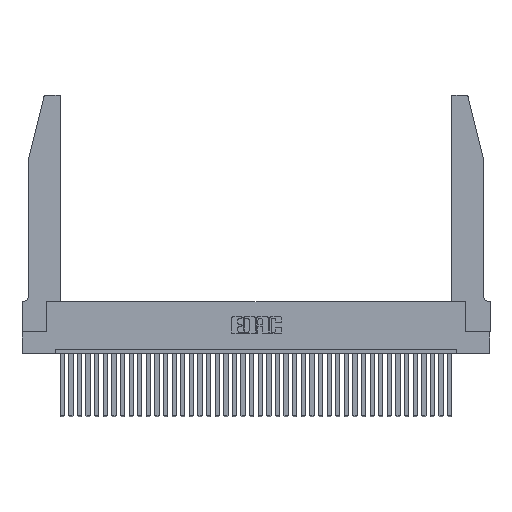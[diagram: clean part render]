
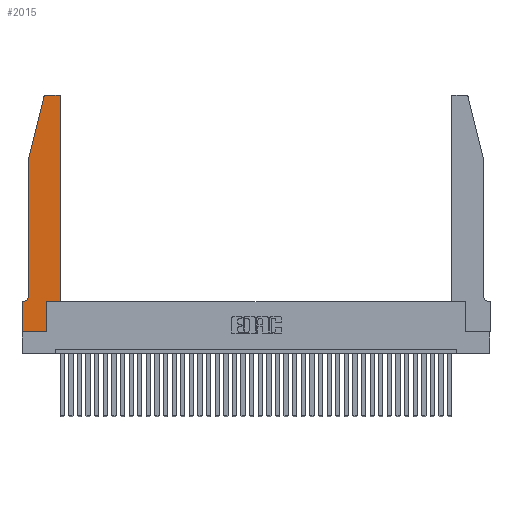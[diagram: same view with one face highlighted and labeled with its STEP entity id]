
A CAD part, top view. The second image highlights one B-rep face of the part: STEP entity #2015.
In plain terms, the highlighted planar face has unit normal (0, 0, 1).
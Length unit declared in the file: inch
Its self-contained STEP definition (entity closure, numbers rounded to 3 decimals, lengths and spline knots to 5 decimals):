
#1285 = DIRECTION ( 'NONE',  ( 0., 1., 0. ) ) ;
#1753 = DIRECTION ( 'NONE',  ( 0., 0., 1. ) ) ;
#1791 = DIRECTION ( 'NONE',  ( 0., 0., 1. ) ) ;
#1822 = EDGE_CURVE ( 'NONE', #13608, #14157, #12460, .T. ) ;
#2015 = ADVANCED_FACE ( 'NONE', ( #34438 ), #25638, .T. ) ;
#2918 = EDGE_CURVE ( 'NONE', #18267, #20375, #23190, .T. ) ;
#3709 = VECTOR ( 'NONE', #16268, 39.37008 ) ;
#4026 = CARTESIAN_POINT ( 'NONE',  ( 0.0755, 0.35, 0.37 ) ) ;
#4498 = DIRECTION ( 'NONE',  ( 1., 0., 0. ) ) ;
#4522 = DIRECTION ( 'NONE',  ( 0., 0., -1. ) ) ;
#5062 = VECTOR ( 'NONE', #18837, 39.37008 ) ;
#5622 = DIRECTION ( 'NONE',  ( 0., -1., 0. ) ) ;
#5947 = EDGE_LOOP ( 'NONE', ( #38282, #24160, #25649, #17477, #10023, #28996, #31484, #28924, #35557, #20605, #14406, #19811 ) ) ;
#6804 = CARTESIAN_POINT ( 'NONE',  ( 0., 0., 0.37 ) ) ;
#6936 = CARTESIAN_POINT ( 'NONE',  ( 0.0755, 2., 0.37 ) ) ;
#7409 = CARTESIAN_POINT ( 'NONE',  ( 0., 0., 0.37 ) ) ;
#7529 = DIRECTION ( 'NONE',  ( -1., 0., 0. ) ) ;
#7593 = DIRECTION ( 'NONE',  ( 0., 1., 0. ) ) ;
#8099 = EDGE_CURVE ( 'NONE', #35104, #13608, #25233, .T. ) ;
#8484 = CARTESIAN_POINT ( 'NONE',  ( 0.4505, 2.72, 0.37 ) ) ;
#9464 = VECTOR ( 'NONE', #1285, 39.37008 ) ;
#9716 = LINE ( 'NONE', #6936, #35869 ) ;
#10023 = ORIENTED_EDGE ( 'NONE', *, *, #11537, .T. ) ;
#10284 = VECTOR ( 'NONE', #16960, 39.37008 ) ;
#10951 = CARTESIAN_POINT ( 'NONE',  ( 0.2605, 2.75, 0.37 ) ) ;
#11537 = EDGE_CURVE ( 'NONE', #20375, #23729, #20236, .T. ) ;
#11818 = VERTEX_POINT ( 'NONE', #37445 ) ;
#12088 = CARTESIAN_POINT ( 'NONE',  ( 0.0755, 0.42, 0.37 ) ) ;
#12460 = LINE ( 'NONE', #6804, #5062 ) ;
#12712 = LINE ( 'NONE', #4026, #26757 ) ;
#13359 = CARTESIAN_POINT ( 'NONE',  ( 0.0055, 0.42, 0.37 ) ) ;
#13608 = VERTEX_POINT ( 'NONE', #33787 ) ;
#13992 = CARTESIAN_POINT ( 'NONE',  ( 0., 0.35, 0.37 ) ) ;
#14157 = VERTEX_POINT ( 'NONE', #16720 ) ;
#14386 = EDGE_CURVE ( 'NONE', #24438, #18267, #9716, .T. ) ;
#14406 = ORIENTED_EDGE ( 'NONE', *, *, #36901, .T. ) ;
#15849 = EDGE_CURVE ( 'NONE', #14157, #19823, #26891, .T. ) ;
#15952 = LINE ( 'NONE', #25290, #9464 ) ;
#16251 = EDGE_CURVE ( 'NONE', #17845, #26636, #37986, .T. ) ;
#16268 = DIRECTION ( 'NONE',  ( 1., 0., 0. ) ) ;
#16474 = DIRECTION ( 'NONE',  ( -0.239, -0.971, 0. ) ) ;
#16720 = CARTESIAN_POINT ( 'NONE',  ( 0.2865, 0., 0.37 ) ) ;
#16960 = DIRECTION ( 'NONE',  ( 0., -1., 0. ) ) ;
#17477 = ORIENTED_EDGE ( 'NONE', *, *, #2918, .T. ) ;
#17845 = VERTEX_POINT ( 'NONE', #8484 ) ;
#18103 = EDGE_CURVE ( 'NONE', #19823, #11818, #18673, .T. ) ;
#18267 = VERTEX_POINT ( 'NONE', #22051 ) ;
#18673 = LINE ( 'NONE', #28291, #3709 ) ;
#18837 = DIRECTION ( 'NONE',  ( 1., 0., 0. ) ) ;
#19685 = CARTESIAN_POINT ( 'NONE',  ( 0.4205, 2.72, 0.37 ) ) ;
#19811 = ORIENTED_EDGE ( 'NONE', *, *, #16251, .T. ) ;
#19823 = VERTEX_POINT ( 'NONE', #34626 ) ;
#19906 = DIRECTION ( 'NONE',  ( 1., 0., 0. ) ) ;
#20236 = CIRCLE ( 'NONE', #37828, 0.07 ) ;
#20375 = VERTEX_POINT ( 'NONE', #12088 ) ;
#20605 = ORIENTED_EDGE ( 'NONE', *, *, #18103, .T. ) ;
#21017 = VECTOR ( 'NONE', #31391, 39.37008 ) ;
#21255 = AXIS2_PLACEMENT_3D ( 'NONE', #37382, #1753, #4498 ) ;
#21536 = CARTESIAN_POINT ( 'NONE',  ( 0., 0.35, 0.37 ) ) ;
#22051 = CARTESIAN_POINT ( 'NONE',  ( 0.0755, 2., 0.37 ) ) ;
#22255 = EDGE_CURVE ( 'NONE', #28313, #24438, #29138, .T. ) ;
#22652 = DIRECTION ( 'NONE',  ( 1., 0., 0. ) ) ;
#23190 = LINE ( 'NONE', #38134, #34352 ) ;
#23515 = EDGE_CURVE ( 'NONE', #26636, #28313, #36440, .T. ) ;
#23729 = VERTEX_POINT ( 'NONE', #35232 ) ;
#24160 = ORIENTED_EDGE ( 'NONE', *, *, #22255, .T. ) ;
#24438 = VERTEX_POINT ( 'NONE', #30622 ) ;
#25233 = LINE ( 'NONE', #7409, #10284 ) ;
#25290 = CARTESIAN_POINT ( 'NONE',  ( 0.4505, 0.35, 0.37 ) ) ;
#25638 = PLANE ( 'NONE',  #32257 ) ;
#25649 = ORIENTED_EDGE ( 'NONE', *, *, #14386, .T. ) ;
#26636 = VERTEX_POINT ( 'NONE', #28118 ) ;
#26757 = VECTOR ( 'NONE', #7529, 39.37008 ) ;
#26891 = LINE ( 'NONE', #28113, #36184 ) ;
#28113 = CARTESIAN_POINT ( 'NONE',  ( 0.2865, 0.35, 0.37 ) ) ;
#28118 = CARTESIAN_POINT ( 'NONE',  ( 0.4205, 2.75, 0.37 ) ) ;
#28126 = CARTESIAN_POINT ( 'NONE',  ( 0.284, 2.75, 0.37 ) ) ;
#28291 = CARTESIAN_POINT ( 'NONE',  ( 0.4505, 0.35, 0.37 ) ) ;
#28313 = VERTEX_POINT ( 'NONE', #28126 ) ;
#28406 = DIRECTION ( 'NONE',  ( -1., 0., 0. ) ) ;
#28924 = ORIENTED_EDGE ( 'NONE', *, *, #1822, .T. ) ;
#28996 = ORIENTED_EDGE ( 'NONE', *, *, #36845, .T. ) ;
#29138 = CIRCLE ( 'NONE', #21255, 0.03 ) ;
#30622 = CARTESIAN_POINT ( 'NONE',  ( 0.25487, 2.72718, 0.37 ) ) ;
#31391 = DIRECTION ( 'NONE',  ( -1., 0., 0. ) ) ;
#31484 = ORIENTED_EDGE ( 'NONE', *, *, #8099, .T. ) ;
#32257 = AXIS2_PLACEMENT_3D ( 'NONE', #13992, #34492, #19906 ) ;
#33787 = CARTESIAN_POINT ( 'NONE',  ( 0., 0., 0.37 ) ) ;
#34352 = VECTOR ( 'NONE', #5622, 39.37008 ) ;
#34438 = FACE_OUTER_BOUND ( 'NONE', #5947, .T. ) ;
#34492 = DIRECTION ( 'NONE',  ( 0., 0., 1. ) ) ;
#34626 = CARTESIAN_POINT ( 'NONE',  ( 0.2865, 0.35, 0.37 ) ) ;
#35104 = VERTEX_POINT ( 'NONE', #21536 ) ;
#35232 = CARTESIAN_POINT ( 'NONE',  ( 0.0055, 0.35, 0.37 ) ) ;
#35557 = ORIENTED_EDGE ( 'NONE', *, *, #15849, .T. ) ;
#35869 = VECTOR ( 'NONE', #16474, 39.37008 ) ;
#36114 = AXIS2_PLACEMENT_3D ( 'NONE', #19685, #1791, #22652 ) ;
#36184 = VECTOR ( 'NONE', #7593, 39.37008 ) ;
#36440 = LINE ( 'NONE', #10951, #21017 ) ;
#36845 = EDGE_CURVE ( 'NONE', #23729, #35104, #12712, .T. ) ;
#36901 = EDGE_CURVE ( 'NONE', #11818, #17845, #15952, .T. ) ;
#37382 = CARTESIAN_POINT ( 'NONE',  ( 0.284, 2.72, 0.37 ) ) ;
#37445 = CARTESIAN_POINT ( 'NONE',  ( 0.4505, 0.35, 0.37 ) ) ;
#37828 = AXIS2_PLACEMENT_3D ( 'NONE', #13359, #4522, #28406 ) ;
#37986 = CIRCLE ( 'NONE', #36114, 0.03 ) ;
#38134 = CARTESIAN_POINT ( 'NONE',  ( 0.0755, 2., 0.37 ) ) ;
#38282 = ORIENTED_EDGE ( 'NONE', *, *, #23515, .T. ) ;
